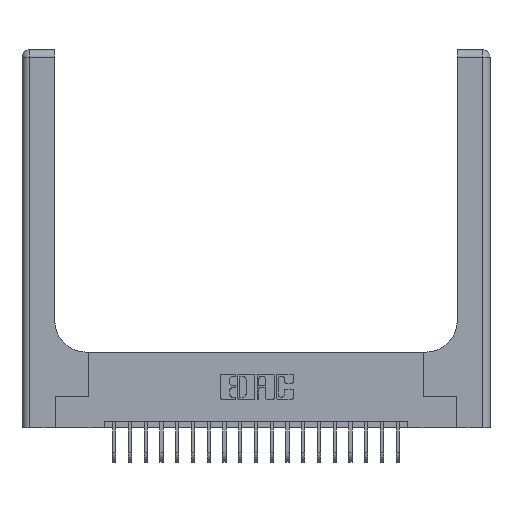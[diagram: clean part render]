
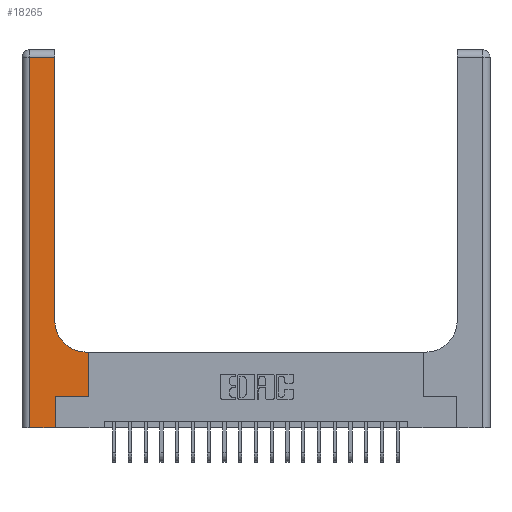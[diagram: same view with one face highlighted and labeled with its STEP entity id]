
A CAD part, top view. The second image highlights one B-rep face of the part: STEP entity #18265.
In plain terms, the highlighted planar face has unit normal (0, 0, 1).
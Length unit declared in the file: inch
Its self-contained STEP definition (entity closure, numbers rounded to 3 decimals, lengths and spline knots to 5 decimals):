
#138 = CARTESIAN_POINT ( 'NONE',  ( 0.51, 0.6, 0.37 ) ) ;
#246 = VERTEX_POINT ( 'NONE', #3221 ) ;
#334 = EDGE_LOOP ( 'NONE', ( #18821, #6429, #12809, #20075, #14960, #13062, #11101, #4029, #6024 ) ) ;
#664 = DIRECTION ( 'NONE',  ( -1., 0., 0. ) ) ;
#686 = CARTESIAN_POINT ( 'NONE',  ( 0.26, 0.85, 0.37 ) ) ;
#719 = PLANE ( 'NONE',  #8047 ) ;
#1334 = VECTOR ( 'NONE', #7269, 39.37008 ) ;
#1468 = VECTOR ( 'NONE', #19643, 39.37008 ) ;
#1538 = DIRECTION ( 'NONE',  ( 0., 1., 0. ) ) ;
#1996 = EDGE_CURVE ( 'NONE', #3064, #9006, #12511, .T. ) ;
#2294 = DIRECTION ( 'NONE',  ( -1., 0., 0. ) ) ;
#2800 = VERTEX_POINT ( 'NONE', #7424 ) ;
#2916 = VECTOR ( 'NONE', #20091, 39.37008 ) ;
#2974 = LINE ( 'NONE', #17595, #10795 ) ;
#3064 = VERTEX_POINT ( 'NONE', #138 ) ;
#3190 = CARTESIAN_POINT ( 'NONE',  ( 0.265, 0.25, 0.37 ) ) ;
#3221 = CARTESIAN_POINT ( 'NONE',  ( 0.265, 0., 0.37 ) ) ;
#3419 = CARTESIAN_POINT ( 'NONE',  ( 0.51, 0.85, 0.37 ) ) ;
#4029 = ORIENTED_EDGE ( 'NONE', *, *, #11734, .T. ) ;
#4991 = DIRECTION ( 'NONE',  ( 1., 0., 0. ) ) ;
#5191 = EDGE_CURVE ( 'NONE', #12972, #2800, #19436, .T. ) ;
#5364 = CARTESIAN_POINT ( 'NONE',  ( 0., 3., 0.37 ) ) ;
#5491 = LINE ( 'NONE', #16584, #1334 ) ;
#5546 = DIRECTION ( 'NONE',  ( 0., 1., 0. ) ) ;
#5641 = LINE ( 'NONE', #14982, #1468 ) ;
#5916 = CARTESIAN_POINT ( 'NONE',  ( 0., 0., 0.37 ) ) ;
#6024 = ORIENTED_EDGE ( 'NONE', *, *, #1996, .T. ) ;
#6429 = ORIENTED_EDGE ( 'NONE', *, *, #17687, .T. ) ;
#6718 = LINE ( 'NONE', #5916, #11327 ) ;
#7040 = VECTOR ( 'NONE', #5546, 39.37008 ) ;
#7269 = DIRECTION ( 'NONE',  ( 1., 0., 0. ) ) ;
#7424 = CARTESIAN_POINT ( 'NONE',  ( 0.528, 0.6, 0.37 ) ) ;
#7949 = CARTESIAN_POINT ( 'NONE',  ( 0.06, 0., 0.37 ) ) ;
#8047 = AXIS2_PLACEMENT_3D ( 'NONE', #5364, #11646, #2294 ) ;
#8749 = VERTEX_POINT ( 'NONE', #7949 ) ;
#9006 = VERTEX_POINT ( 'NONE', #686 ) ;
#9037 = VECTOR ( 'NONE', #1538, 39.37008 ) ;
#9791 = DIRECTION ( 'NONE',  ( -1., 0., 0. ) ) ;
#10005 = CARTESIAN_POINT ( 'NONE',  ( 0., 2.94, 0.37 ) ) ;
#10242 = EDGE_CURVE ( 'NONE', #8749, #246, #6718, .T. ) ;
#10795 = VECTOR ( 'NONE', #9791, 39.37008 ) ;
#11101 = ORIENTED_EDGE ( 'NONE', *, *, #5191, .T. ) ;
#11223 = LINE ( 'NONE', #12394, #2916 ) ;
#11317 = VECTOR ( 'NONE', #664, 39.37008 ) ;
#11327 = VECTOR ( 'NONE', #18360, 39.37008 ) ;
#11539 = VERTEX_POINT ( 'NONE', #3190 ) ;
#11646 = DIRECTION ( 'NONE',  ( 0., 0., -1. ) ) ;
#11734 = EDGE_CURVE ( 'NONE', #2800, #3064, #2974, .T. ) ;
#12394 = CARTESIAN_POINT ( 'NONE',  ( 0.06, 3., 0.37 ) ) ;
#12511 = CIRCLE ( 'NONE', #16832, 0.25 ) ;
#12809 = ORIENTED_EDGE ( 'NONE', *, *, #13506, .T. ) ;
#12972 = VERTEX_POINT ( 'NONE', #14525 ) ;
#13062 = ORIENTED_EDGE ( 'NONE', *, *, #17180, .T. ) ;
#13506 = EDGE_CURVE ( 'NONE', #17712, #8749, #11223, .T. ) ;
#13673 = LINE ( 'NONE', #20162, #9037 ) ;
#14349 = DIRECTION ( 'NONE',  ( 0., 0., -1. ) ) ;
#14466 = FACE_OUTER_BOUND ( 'NONE', #334, .T. ) ;
#14525 = CARTESIAN_POINT ( 'NONE',  ( 0.528, 0.25, 0.37 ) ) ;
#14960 = ORIENTED_EDGE ( 'NONE', *, *, #19670, .T. ) ;
#14982 = CARTESIAN_POINT ( 'NONE',  ( 0.265, 0., 0.37 ) ) ;
#16210 = VERTEX_POINT ( 'NONE', #17280 ) ;
#16449 = CARTESIAN_POINT ( 'NONE',  ( 0.528, 0.25, 0.37 ) ) ;
#16584 = CARTESIAN_POINT ( 'NONE',  ( 0.265, 0.25, 0.37 ) ) ;
#16832 = AXIS2_PLACEMENT_3D ( 'NONE', #3419, #14349, #4991 ) ;
#17180 = EDGE_CURVE ( 'NONE', #11539, #12972, #5491, .T. ) ;
#17280 = CARTESIAN_POINT ( 'NONE',  ( 0.26, 2.94, 0.37 ) ) ;
#17595 = CARTESIAN_POINT ( 'NONE',  ( 0.26, 0.6, 0.37 ) ) ;
#17687 = EDGE_CURVE ( 'NONE', #16210, #17712, #19571, .T. ) ;
#17712 = VERTEX_POINT ( 'NONE', #17858 ) ;
#17858 = CARTESIAN_POINT ( 'NONE',  ( 0.06, 2.94, 0.37 ) ) ;
#18265 = ADVANCED_FACE ( 'NONE', ( #14466 ), #719, .F. ) ;
#18360 = DIRECTION ( 'NONE',  ( 1., 0., 0. ) ) ;
#18821 = ORIENTED_EDGE ( 'NONE', *, *, #19905, .T. ) ;
#19436 = LINE ( 'NONE', #16449, #7040 ) ;
#19571 = LINE ( 'NONE', #10005, #11317 ) ;
#19643 = DIRECTION ( 'NONE',  ( 0., 1., 0. ) ) ;
#19670 = EDGE_CURVE ( 'NONE', #246, #11539, #5641, .T. ) ;
#19905 = EDGE_CURVE ( 'NONE', #9006, #16210, #13673, .T. ) ;
#20075 = ORIENTED_EDGE ( 'NONE', *, *, #10242, .T. ) ;
#20091 = DIRECTION ( 'NONE',  ( 0., -1., 0. ) ) ;
#20162 = CARTESIAN_POINT ( 'NONE',  ( 0.26, 3., 0.37 ) ) ;
